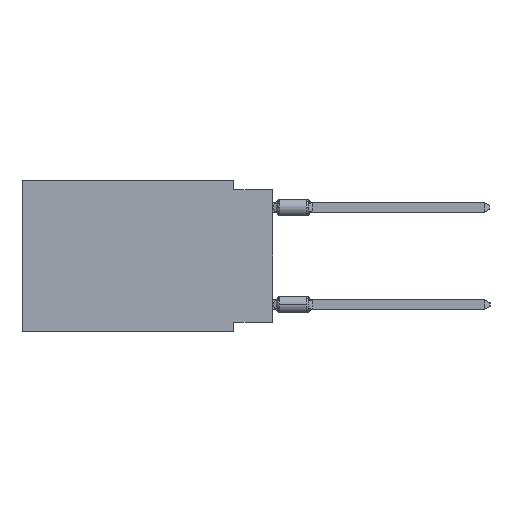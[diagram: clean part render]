
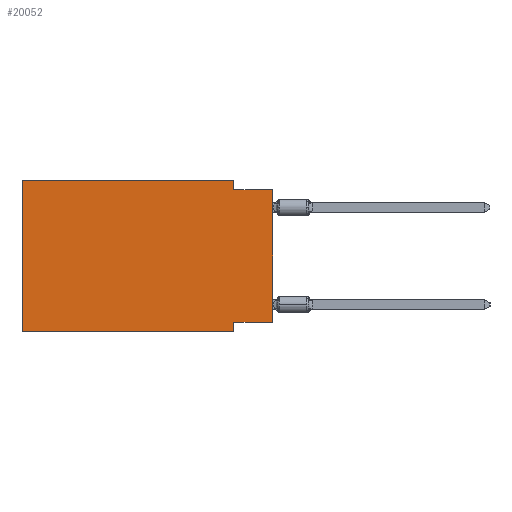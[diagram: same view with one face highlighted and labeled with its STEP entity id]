
A CAD part, left-side view. The second image highlights one B-rep face of the part: STEP entity #20052.
In plain terms, the highlighted planar face has unit normal (-1, 0, 0).
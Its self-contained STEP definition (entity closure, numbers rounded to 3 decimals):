
#479 = VECTOR ( 'NONE', #32973, 1000. ) ;
#705 = DIRECTION ( 'NONE',  ( 0., 0., -1. ) ) ;
#2098 = DIRECTION ( 'NONE',  ( 0., 0., -1. ) ) ;
#2937 = ORIENTED_EDGE ( 'NONE', *, *, #46562, .F. ) ;
#2964 = EDGE_CURVE ( 'NONE', #17285, #27511, #46146, .T. ) ;
#3398 = LINE ( 'NONE', #35169, #41771 ) ;
#3901 = CARTESIAN_POINT ( 'NONE',  ( 0., 2.54, -9.271 ) ) ;
#5398 = LINE ( 'NONE', #10498, #36922 ) ;
#6294 = CARTESIAN_POINT ( 'NONE',  ( 0., 16.383, 0. ) ) ;
#6375 = CARTESIAN_POINT ( 'NONE',  ( 0., 2.54, 0. ) ) ;
#7735 = ORIENTED_EDGE ( 'NONE', *, *, #22929, .F. ) ;
#7950 = CARTESIAN_POINT ( 'NONE',  ( 0., 0., -9.271 ) ) ;
#8410 = AXIS2_PLACEMENT_3D ( 'NONE', #6294, #42855, #2098 ) ;
#8602 = VECTOR ( 'NONE', #50062, 1000. ) ;
#8849 = VERTEX_POINT ( 'NONE', #54831 ) ;
#10058 = VERTEX_POINT ( 'NONE', #11381 ) ;
#10498 = CARTESIAN_POINT ( 'NONE',  ( 0., 16.383, 0. ) ) ;
#11330 = EDGE_CURVE ( 'NONE', #19441, #10058, #33938, .T. ) ;
#11381 = CARTESIAN_POINT ( 'NONE',  ( 0., 2.54, -0.635 ) ) ;
#14118 = VERTEX_POINT ( 'NONE', #18432 ) ;
#14692 = CARTESIAN_POINT ( 'NONE',  ( 0., 0., -0.635 ) ) ;
#14895 = CARTESIAN_POINT ( 'NONE',  ( 0., 16.383, 0. ) ) ;
#14915 = EDGE_CURVE ( 'NONE', #8849, #14118, #26341, .T. ) ;
#16446 = PLANE ( 'NONE',  #8410 ) ;
#16691 = ORIENTED_EDGE ( 'NONE', *, *, #2964, .T. ) ;
#17285 = VERTEX_POINT ( 'NONE', #47131 ) ;
#18432 = CARTESIAN_POINT ( 'NONE',  ( 0., 2.54, -9.906 ) ) ;
#18994 = VECTOR ( 'NONE', #24770, 1000. ) ;
#19174 = LINE ( 'NONE', #14692, #479 ) ;
#19441 = VERTEX_POINT ( 'NONE', #28830 ) ;
#20010 = EDGE_LOOP ( 'NONE', ( #16691, #31308, #38299, #7735, #35448, #40262, #51106, #2937 ) ) ;
#20052 = ADVANCED_FACE ( 'NONE', ( #57513 ), #16446, .F. ) ;
#22489 = CARTESIAN_POINT ( 'NONE',  ( 0., 0., 0. ) ) ;
#22929 = EDGE_CURVE ( 'NONE', #51583, #19441, #3398, .T. ) ;
#24103 = EDGE_CURVE ( 'NONE', #47530, #14118, #30744, .T. ) ;
#24770 = DIRECTION ( 'NONE',  ( 0., 0., -1. ) ) ;
#26341 = LINE ( 'NONE', #53913, #31814 ) ;
#27511 = VERTEX_POINT ( 'NONE', #47979 ) ;
#28830 = CARTESIAN_POINT ( 'NONE',  ( 0., 2.54, 0. ) ) ;
#29726 = VECTOR ( 'NONE', #705, 1000. ) ;
#30744 = LINE ( 'NONE', #53219, #18994 ) ;
#31308 = ORIENTED_EDGE ( 'NONE', *, *, #33044, .F. ) ;
#31814 = VECTOR ( 'NONE', #44610, 1000. ) ;
#32973 = DIRECTION ( 'NONE',  ( 0., -1., 0. ) ) ;
#33044 = EDGE_CURVE ( 'NONE', #10058, #27511, #19174, .T. ) ;
#33938 = LINE ( 'NONE', #6375, #29726 ) ;
#34571 = DIRECTION ( 'NONE',  ( 0., -1., 0. ) ) ;
#35169 = CARTESIAN_POINT ( 'NONE',  ( 0., 16.383, 0. ) ) ;
#35448 = ORIENTED_EDGE ( 'NONE', *, *, #52744, .F. ) ;
#36922 = VECTOR ( 'NONE', #51541, 1000. ) ;
#38299 = ORIENTED_EDGE ( 'NONE', *, *, #11330, .F. ) ;
#40262 = ORIENTED_EDGE ( 'NONE', *, *, #14915, .T. ) ;
#41771 = VECTOR ( 'NONE', #34571, 1000. ) ;
#42855 = DIRECTION ( 'NONE',  ( 1., 0., 0. ) ) ;
#44610 = DIRECTION ( 'NONE',  ( 0., -1., 0. ) ) ;
#46146 = LINE ( 'NONE', #22489, #8602 ) ;
#46562 = EDGE_CURVE ( 'NONE', #17285, #47530, #53487, .T. ) ;
#47131 = CARTESIAN_POINT ( 'NONE',  ( 0., 0., -9.271 ) ) ;
#47530 = VERTEX_POINT ( 'NONE', #3901 ) ;
#47979 = CARTESIAN_POINT ( 'NONE',  ( 0., 0., -0.635 ) ) ;
#50062 = DIRECTION ( 'NONE',  ( 0., 0., 1. ) ) ;
#50884 = VECTOR ( 'NONE', #57985, 1000. ) ;
#51106 = ORIENTED_EDGE ( 'NONE', *, *, #24103, .F. ) ;
#51541 = DIRECTION ( 'NONE',  ( 0., 0., 1. ) ) ;
#51583 = VERTEX_POINT ( 'NONE', #14895 ) ;
#52744 = EDGE_CURVE ( 'NONE', #8849, #51583, #5398, .T. ) ;
#53219 = CARTESIAN_POINT ( 'NONE',  ( 0., 2.54, -9.906 ) ) ;
#53487 = LINE ( 'NONE', #7950, #50884 ) ;
#53913 = CARTESIAN_POINT ( 'NONE',  ( 0., 16.383, -9.906 ) ) ;
#54831 = CARTESIAN_POINT ( 'NONE',  ( 0., 16.383, -9.906 ) ) ;
#57513 = FACE_OUTER_BOUND ( 'NONE', #20010, .T. ) ;
#57985 = DIRECTION ( 'NONE',  ( 0., 1., 0. ) ) ;
